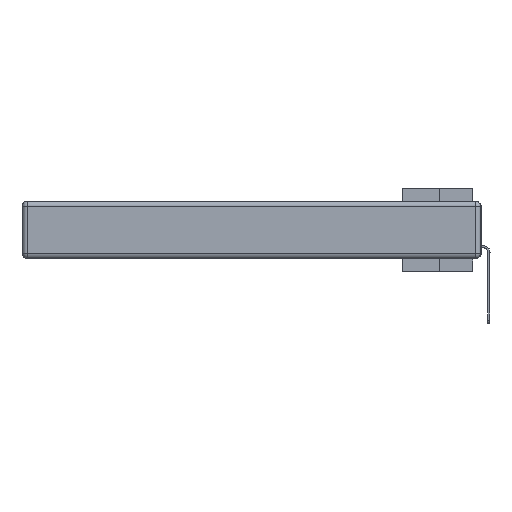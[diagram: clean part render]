
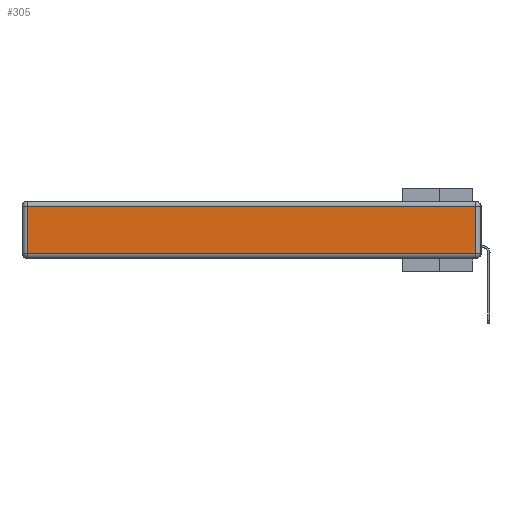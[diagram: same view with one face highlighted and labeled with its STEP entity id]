
A CAD part, left-side view. The second image highlights one B-rep face of the part: STEP entity #305.
In plain terms, the highlighted planar face has unit normal (-1, 0, 0).
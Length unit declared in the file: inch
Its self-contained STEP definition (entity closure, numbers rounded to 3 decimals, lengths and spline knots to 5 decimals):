
#305 = ADVANCED_FACE ( 'NONE', ( #37241 ), #37440, .T. ) ;
#3207 = AXIS2_PLACEMENT_3D ( 'NONE', #22189, #16977, #19691 ) ;
#3834 = CARTESIAN_POINT ( 'NONE',  ( 0., 2.72, -0.343 ) ) ;
#4621 = DIRECTION ( 'NONE',  ( 0., 0., -1. ) ) ;
#5479 = ORIENTED_EDGE ( 'NONE', *, *, #27745, .T. ) ;
#5553 = VECTOR ( 'NONE', #4621, 39.37008 ) ;
#5562 = CARTESIAN_POINT ( 'NONE',  ( 0., 0., -0.313 ) ) ;
#6368 = CARTESIAN_POINT ( 'NONE',  ( 0., 2.75, -0.03 ) ) ;
#6379 = ORIENTED_EDGE ( 'NONE', *, *, #15217, .T. ) ;
#6880 = CARTESIAN_POINT ( 'NONE',  ( 0., 0.03, -0.313 ) ) ;
#8724 = ORIENTED_EDGE ( 'NONE', *, *, #20295, .T. ) ;
#9375 = CARTESIAN_POINT ( 'NONE',  ( 0., 2.72, -0.03 ) ) ;
#11755 = VERTEX_POINT ( 'NONE', #9375 ) ;
#12809 = VERTEX_POINT ( 'NONE', #6880 ) ;
#13638 = DIRECTION ( 'NONE',  ( 0., 0., 1. ) ) ;
#15217 = EDGE_CURVE ( 'NONE', #26811, #11755, #32815, .T. ) ;
#16977 = DIRECTION ( 'NONE',  ( -1., 0., 0. ) ) ;
#17511 = LINE ( 'NONE', #5562, #27586 ) ;
#19691 = DIRECTION ( 'NONE',  ( 0., 0., 1. ) ) ;
#20295 = EDGE_CURVE ( 'NONE', #11755, #30306, #24693, .T. ) ;
#20806 = EDGE_LOOP ( 'NONE', ( #27893, #5479, #6379, #8724 ) ) ;
#22189 = CARTESIAN_POINT ( 'NONE',  ( 0., 0., -0.343 ) ) ;
#24693 = LINE ( 'NONE', #3834, #5553 ) ;
#26811 = VERTEX_POINT ( 'NONE', #34054 ) ;
#27020 = DIRECTION ( 'NONE',  ( 0., 1., 0. ) ) ;
#27586 = VECTOR ( 'NONE', #32191, 39.37008 ) ;
#27745 = EDGE_CURVE ( 'NONE', #12809, #26811, #34502, .T. ) ;
#27893 = ORIENTED_EDGE ( 'NONE', *, *, #32866, .T. ) ;
#29217 = VECTOR ( 'NONE', #13638, 39.37008 ) ;
#30306 = VERTEX_POINT ( 'NONE', #37199 ) ;
#31027 = CARTESIAN_POINT ( 'NONE',  ( 0., 0.03, -0.343 ) ) ;
#32191 = DIRECTION ( 'NONE',  ( 0., -1., 0. ) ) ;
#32815 = LINE ( 'NONE', #6368, #33593 ) ;
#32866 = EDGE_CURVE ( 'NONE', #30306, #12809, #17511, .T. ) ;
#33593 = VECTOR ( 'NONE', #27020, 39.37008 ) ;
#34054 = CARTESIAN_POINT ( 'NONE',  ( 0., 0.03, -0.03 ) ) ;
#34502 = LINE ( 'NONE', #31027, #29217 ) ;
#37199 = CARTESIAN_POINT ( 'NONE',  ( 0., 2.72, -0.313 ) ) ;
#37241 = FACE_OUTER_BOUND ( 'NONE', #20806, .T. ) ;
#37440 = PLANE ( 'NONE',  #3207 ) ;
